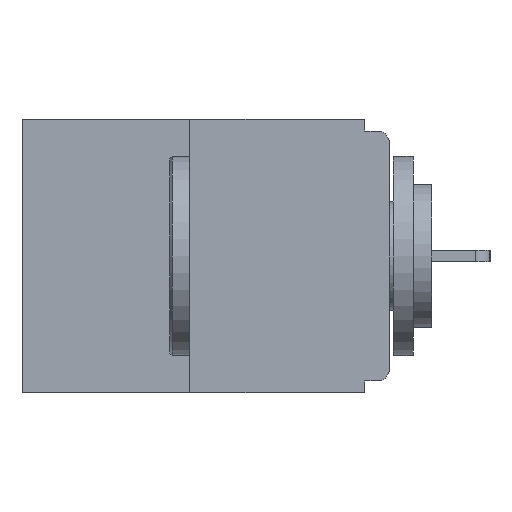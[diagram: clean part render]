
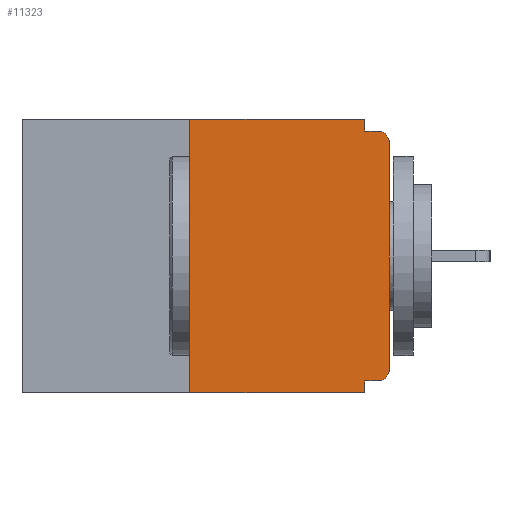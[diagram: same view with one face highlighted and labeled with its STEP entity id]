
A CAD part, left-side view. The second image highlights one B-rep face of the part: STEP entity #11323.
In plain terms, the highlighted planar face has unit normal (-1, 0, 0).
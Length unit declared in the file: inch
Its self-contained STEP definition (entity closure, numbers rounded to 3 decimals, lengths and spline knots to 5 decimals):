
#54 = DIRECTION ( 'NONE',  ( 0., 0., -1. ) ) ;
#104 = EDGE_CURVE ( 'NONE', #6170, #10477, #8045, .T. ) ;
#174 = LINE ( 'NONE', #10328, #11384 ) ;
#261 = EDGE_CURVE ( 'NONE', #8226, #10349, #9048, .T. ) ;
#411 = CARTESIAN_POINT ( 'NONE',  ( 0., 0., 0. ) ) ;
#440 = DIRECTION ( 'NONE',  ( -1., 0., 0. ) ) ;
#575 = PLANE ( 'NONE',  #10008 ) ;
#703 = DIRECTION ( 'NONE',  ( 0., -1., 0. ) ) ;
#750 = DIRECTION ( 'NONE',  ( 0., 0., -1. ) ) ;
#849 = CARTESIAN_POINT ( 'NONE',  ( 0., 0.015, -0.313 ) ) ;
#906 = DIRECTION ( 'NONE',  ( -1., 0., 0. ) ) ;
#1200 = VECTOR ( 'NONE', #5050, 39.37008 ) ;
#1250 = ORIENTED_EDGE ( 'NONE', *, *, #9547, .F. ) ;
#1317 = CIRCLE ( 'NONE', #1514, 0.015 ) ;
#1322 = LINE ( 'NONE', #2201, #4601 ) ;
#1488 = CARTESIAN_POINT ( 'NONE',  ( 0., 0.031, -0.328 ) ) ;
#1514 = AXIS2_PLACEMENT_3D ( 'NONE', #849, #906, #8390 ) ;
#1681 = VERTEX_POINT ( 'NONE', #1488 ) ;
#1842 = CARTESIAN_POINT ( 'NONE',  ( 0., 0.46, -0.343 ) ) ;
#2055 = VERTEX_POINT ( 'NONE', #2564 ) ;
#2072 = ORIENTED_EDGE ( 'NONE', *, *, #3983, .T. ) ;
#2201 = CARTESIAN_POINT ( 'NONE',  ( 0., 0.25, 0. ) ) ;
#2564 = CARTESIAN_POINT ( 'NONE',  ( 0., 0., -0.313 ) ) ;
#2675 = DIRECTION ( 'NONE',  ( 1., 0., 0. ) ) ;
#2685 = VECTOR ( 'NONE', #8388, 39.37008 ) ;
#2696 = CARTESIAN_POINT ( 'NONE',  ( 0., 0., -0.03 ) ) ;
#3175 = VERTEX_POINT ( 'NONE', #7100 ) ;
#3410 = EDGE_CURVE ( 'NONE', #5574, #2055, #1317, .T. ) ;
#3518 = CARTESIAN_POINT ( 'NONE',  ( 0., 0.015, -0.328 ) ) ;
#3525 = EDGE_CURVE ( 'NONE', #3175, #6657, #1322, .T. ) ;
#3620 = ORIENTED_EDGE ( 'NONE', *, *, #3971, .F. ) ;
#3623 = VERTEX_POINT ( 'NONE', #9857 ) ;
#3971 = EDGE_CURVE ( 'NONE', #5574, #1681, #4065, .T. ) ;
#3983 = EDGE_CURVE ( 'NONE', #3175, #3623, #10327, .T. ) ;
#4065 = LINE ( 'NONE', #5518, #8902 ) ;
#4203 = VECTOR ( 'NONE', #9641, 39.37008 ) ;
#4601 = VECTOR ( 'NONE', #5137, 39.37008 ) ;
#4679 = ORIENTED_EDGE ( 'NONE', *, *, #6824, .F. ) ;
#4783 = DIRECTION ( 'NONE',  ( 0., -1., 0. ) ) ;
#4861 = CARTESIAN_POINT ( 'NONE',  ( 0., 0.015, -0.03 ) ) ;
#5039 = DIRECTION ( 'NONE',  ( 0., 0., -1. ) ) ;
#5050 = DIRECTION ( 'NONE',  ( 0., 0., -1. ) ) ;
#5137 = DIRECTION ( 'NONE',  ( 0., 0., 1. ) ) ;
#5430 = ORIENTED_EDGE ( 'NONE', *, *, #3525, .F. ) ;
#5518 = CARTESIAN_POINT ( 'NONE',  ( 0., 0., -0.328 ) ) ;
#5574 = VERTEX_POINT ( 'NONE', #3518 ) ;
#5664 = ORIENTED_EDGE ( 'NONE', *, *, #12009, .T. ) ;
#6170 = VERTEX_POINT ( 'NONE', #2696 ) ;
#6219 = LINE ( 'NONE', #11763, #1200 ) ;
#6435 = CARTESIAN_POINT ( 'NONE',  ( 0., 0.031, -0.015 ) ) ;
#6625 = CARTESIAN_POINT ( 'NONE',  ( 0., 0.031, 0. ) ) ;
#6657 = VERTEX_POINT ( 'NONE', #11184 ) ;
#6770 = EDGE_LOOP ( 'NONE', ( #1250, #5430, #2072, #4679, #3620, #8685, #5664, #11809, #8214, #8977 ) ) ;
#6824 = EDGE_CURVE ( 'NONE', #1681, #3623, #6219, .T. ) ;
#7074 = CARTESIAN_POINT ( 'NONE',  ( 0., 0.46, 0. ) ) ;
#7100 = CARTESIAN_POINT ( 'NONE',  ( 0., 0.25, -0.343 ) ) ;
#7261 = VECTOR ( 'NONE', #54, 39.37008 ) ;
#8045 = CIRCLE ( 'NONE', #9570, 0.015 ) ;
#8105 = DIRECTION ( 'NONE',  ( 0., 1., 0. ) ) ;
#8214 = ORIENTED_EDGE ( 'NONE', *, *, #10038, .F. ) ;
#8226 = VERTEX_POINT ( 'NONE', #11939 ) ;
#8388 = DIRECTION ( 'NONE',  ( 0., -1., 0. ) ) ;
#8390 = DIRECTION ( 'NONE',  ( 0., 0., -1. ) ) ;
#8435 = CARTESIAN_POINT ( 'NONE',  ( 0., 0.015, -0.015 ) ) ;
#8631 = VECTOR ( 'NONE', #703, 39.37008 ) ;
#8685 = ORIENTED_EDGE ( 'NONE', *, *, #3410, .T. ) ;
#8902 = VECTOR ( 'NONE', #8105, 39.37008 ) ;
#8954 = FACE_OUTER_BOUND ( 'NONE', #6770, .T. ) ;
#8977 = ORIENTED_EDGE ( 'NONE', *, *, #261, .F. ) ;
#9048 = LINE ( 'NONE', #6625, #7261 ) ;
#9199 = LINE ( 'NONE', #10904, #8631 ) ;
#9547 = EDGE_CURVE ( 'NONE', #6657, #8226, #9199, .T. ) ;
#9570 = AXIS2_PLACEMENT_3D ( 'NONE', #4861, #440, #5039 ) ;
#9641 = DIRECTION ( 'NONE',  ( 0., 0., 1. ) ) ;
#9857 = CARTESIAN_POINT ( 'NONE',  ( 0., 0.031, -0.343 ) ) ;
#10008 = AXIS2_PLACEMENT_3D ( 'NONE', #7074, #2675, #750 ) ;
#10038 = EDGE_CURVE ( 'NONE', #10349, #10477, #174, .T. ) ;
#10327 = LINE ( 'NONE', #1842, #2685 ) ;
#10328 = CARTESIAN_POINT ( 'NONE',  ( 0., 0., -0.015 ) ) ;
#10349 = VERTEX_POINT ( 'NONE', #6435 ) ;
#10477 = VERTEX_POINT ( 'NONE', #8435 ) ;
#10904 = CARTESIAN_POINT ( 'NONE',  ( 0., 0.46, 0. ) ) ;
#11184 = CARTESIAN_POINT ( 'NONE',  ( 0., 0.25, 0. ) ) ;
#11323 = ADVANCED_FACE ( 'NONE', ( #8954 ), #575, .F. ) ;
#11384 = VECTOR ( 'NONE', #4783, 39.37008 ) ;
#11729 = LINE ( 'NONE', #411, #4203 ) ;
#11763 = CARTESIAN_POINT ( 'NONE',  ( 0., 0.031, -0.343 ) ) ;
#11809 = ORIENTED_EDGE ( 'NONE', *, *, #104, .T. ) ;
#11939 = CARTESIAN_POINT ( 'NONE',  ( 0., 0.031, 0. ) ) ;
#12009 = EDGE_CURVE ( 'NONE', #2055, #6170, #11729, .T. ) ;
